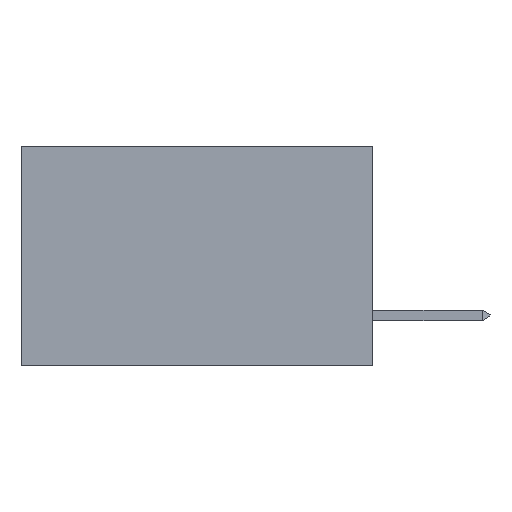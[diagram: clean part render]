
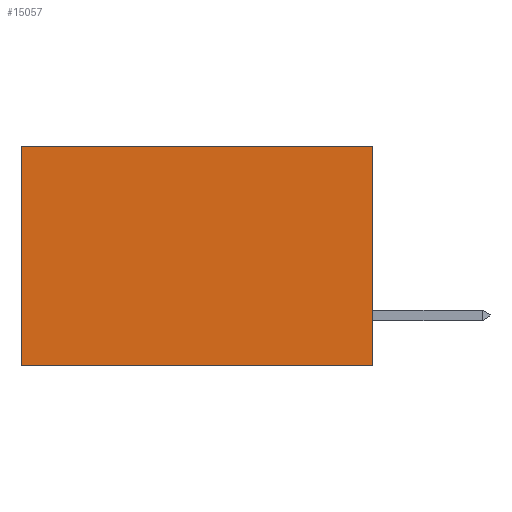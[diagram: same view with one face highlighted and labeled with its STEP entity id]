
A CAD part, left-side view. The second image highlights one B-rep face of the part: STEP entity #15057.
In plain terms, the highlighted planar face has unit normal (-1, 0, 0).
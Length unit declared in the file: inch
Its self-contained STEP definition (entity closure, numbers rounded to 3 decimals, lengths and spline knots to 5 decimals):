
#84 = CARTESIAN_POINT ( 'NONE',  ( 0.277, 0., -0.37 ) ) ;
#1955 = EDGE_CURVE ( 'NONE', #4680, #2332, #13289, .T. ) ;
#2133 = DIRECTION ( 'NONE',  ( 0., 0., -1. ) ) ;
#2301 = CARTESIAN_POINT ( 'NONE',  ( 0.277, 0.59, -0.37 ) ) ;
#2332 = VERTEX_POINT ( 'NONE', #8875 ) ;
#2358 = CARTESIAN_POINT ( 'NONE',  ( 0.277, 0., 0. ) ) ;
#2583 = ORIENTED_EDGE ( 'NONE', *, *, #7950, .T. ) ;
#3588 = VECTOR ( 'NONE', #2133, 39.37008 ) ;
#3678 = ORIENTED_EDGE ( 'NONE', *, *, #14587, .T. ) ;
#4665 = CARTESIAN_POINT ( 'NONE',  ( 0.277, 0.59, -0.37 ) ) ;
#4680 = VERTEX_POINT ( 'NONE', #6810 ) ;
#5354 = LINE ( 'NONE', #2358, #18693 ) ;
#5434 = PLANE ( 'NONE',  #8800 ) ;
#6810 = CARTESIAN_POINT ( 'NONE',  ( 0.277, 0., 0. ) ) ;
#7874 = ORIENTED_EDGE ( 'NONE', *, *, #1955, .F. ) ;
#7950 = EDGE_CURVE ( 'NONE', #12952, #10334, #9995, .T. ) ;
#8126 = VECTOR ( 'NONE', #15379, 39.37008 ) ;
#8655 = VECTOR ( 'NONE', #12086, 39.37008 ) ;
#8800 = AXIS2_PLACEMENT_3D ( 'NONE', #84, #19342, #9007 ) ;
#8875 = CARTESIAN_POINT ( 'NONE',  ( 0.277, 0., -0.37 ) ) ;
#8952 = FACE_OUTER_BOUND ( 'NONE', #13215, .T. ) ;
#9007 = DIRECTION ( 'NONE',  ( 0., 0., -1. ) ) ;
#9995 = LINE ( 'NONE', #2301, #3588 ) ;
#10334 = VERTEX_POINT ( 'NONE', #4665 ) ;
#12086 = DIRECTION ( 'NONE',  ( 0., 0., -1. ) ) ;
#12952 = VERTEX_POINT ( 'NONE', #17538 ) ;
#13215 = EDGE_LOOP ( 'NONE', ( #2583, #16540, #7874, #3678 ) ) ;
#13289 = LINE ( 'NONE', #14030, #8655 ) ;
#13669 = CARTESIAN_POINT ( 'NONE',  ( 0.277, 0., -0.37 ) ) ;
#14030 = CARTESIAN_POINT ( 'NONE',  ( 0.277, 0., -0.37 ) ) ;
#14587 = EDGE_CURVE ( 'NONE', #4680, #12952, #5354, .T. ) ;
#14878 = EDGE_CURVE ( 'NONE', #2332, #10334, #17331, .T. ) ;
#15057 = ADVANCED_FACE ( 'NONE', ( #8952 ), #5434, .F. ) ;
#15379 = DIRECTION ( 'NONE',  ( 0., 1., 0. ) ) ;
#16280 = DIRECTION ( 'NONE',  ( 0., 1., 0. ) ) ;
#16540 = ORIENTED_EDGE ( 'NONE', *, *, #14878, .F. ) ;
#17331 = LINE ( 'NONE', #13669, #8126 ) ;
#17538 = CARTESIAN_POINT ( 'NONE',  ( 0.277, 0.59, 0. ) ) ;
#18693 = VECTOR ( 'NONE', #16280, 39.37008 ) ;
#19342 = DIRECTION ( 'NONE',  ( 1., 0., 0. ) ) ;
